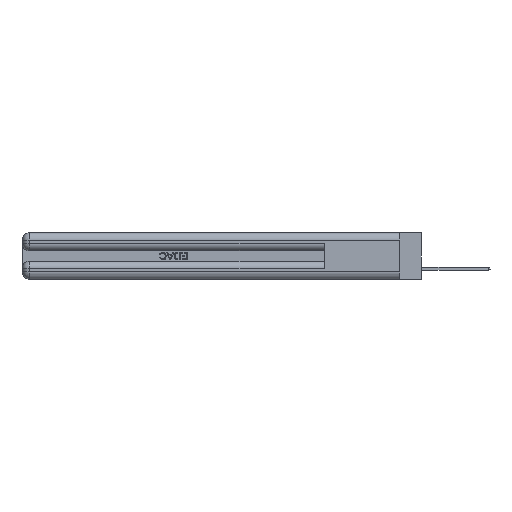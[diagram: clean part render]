
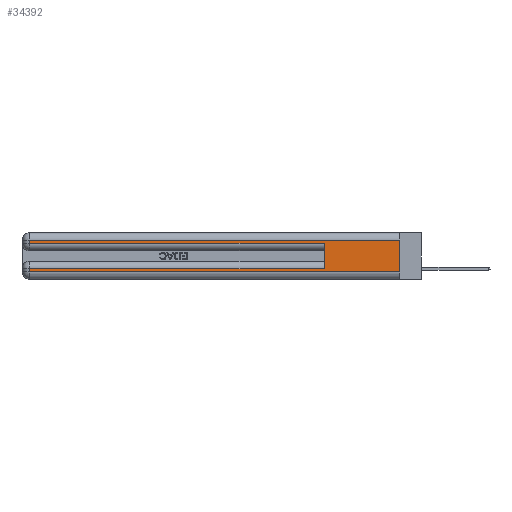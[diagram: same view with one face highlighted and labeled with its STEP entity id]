
A CAD part, left-side view. The second image highlights one B-rep face of the part: STEP entity #34392.
In plain terms, the highlighted planar face has unit normal (-1, 0, 0).
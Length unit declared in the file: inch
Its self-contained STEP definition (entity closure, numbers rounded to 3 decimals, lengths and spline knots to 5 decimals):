
#2489 = LINE ( 'NONE', #6364, #8938 ) ;
#2717 = VERTEX_POINT ( 'NONE', #44504 ) ;
#3348 = CARTESIAN_POINT ( 'NONE',  ( 0., 0.6, 0.085 ) ) ;
#4973 = CARTESIAN_POINT ( 'NONE',  ( 0., 2.94, 0.31 ) ) ;
#5919 = VECTOR ( 'NONE', #8321, 39.37008 ) ;
#6348 = ORIENTED_EDGE ( 'NONE', *, *, #17489, .T. ) ;
#6364 = CARTESIAN_POINT ( 'NONE',  ( 0., 0., 0.285 ) ) ;
#8077 = LINE ( 'NONE', #38608, #26345 ) ;
#8116 = CARTESIAN_POINT ( 'NONE',  ( 0., 0., 0.31 ) ) ;
#8321 = DIRECTION ( 'NONE',  ( 0., 0., 1. ) ) ;
#8938 = VECTOR ( 'NONE', #42705, 39.37008 ) ;
#9776 = LINE ( 'NONE', #14755, #48023 ) ;
#10958 = CARTESIAN_POINT ( 'NONE',  ( 0., 2.94, 0.085 ) ) ;
#11423 = LINE ( 'NONE', #25829, #29112 ) ;
#11937 = CARTESIAN_POINT ( 'NONE',  ( 0., 0.6, 0.145 ) ) ;
#12087 = PLANE ( 'NONE',  #47939 ) ;
#12150 = VERTEX_POINT ( 'NONE', #16853 ) ;
#12920 = DIRECTION ( 'NONE',  ( 0., 0., -1. ) ) ;
#13185 = EDGE_CURVE ( 'NONE', #21291, #37837, #46464, .T. ) ;
#13463 = CARTESIAN_POINT ( 'NONE',  ( 0., 0., 0.06 ) ) ;
#14755 = CARTESIAN_POINT ( 'NONE',  ( 0., 0., 0.37 ) ) ;
#15212 = CARTESIAN_POINT ( 'NONE',  ( 0., 0., 0.06 ) ) ;
#15460 = LINE ( 'NONE', #15524, #24281 ) ;
#15524 = CARTESIAN_POINT ( 'NONE',  ( 0., 0., 0.085 ) ) ;
#15884 = ORIENTED_EDGE ( 'NONE', *, *, #40547, .F. ) ;
#16217 = EDGE_CURVE ( 'NONE', #18066, #12150, #38505, .T. ) ;
#16572 = ORIENTED_EDGE ( 'NONE', *, *, #46242, .T. ) ;
#16853 = CARTESIAN_POINT ( 'NONE',  ( 0., 2.94, 0.06 ) ) ;
#17173 = ORIENTED_EDGE ( 'NONE', *, *, #16217, .T. ) ;
#17489 = EDGE_CURVE ( 'NONE', #2717, #37837, #2489, .T. ) ;
#18066 = VERTEX_POINT ( 'NONE', #10958 ) ;
#18533 = VECTOR ( 'NONE', #43790, 39.37008 ) ;
#21291 = VERTEX_POINT ( 'NONE', #3348 ) ;
#24074 = DIRECTION ( 'NONE',  ( 1., 0., 0. ) ) ;
#24281 = VECTOR ( 'NONE', #45780, 39.37008 ) ;
#24666 = ORIENTED_EDGE ( 'NONE', *, *, #13185, .F. ) ;
#25829 = CARTESIAN_POINT ( 'NONE',  ( 0., 2.94, 0.37 ) ) ;
#25979 = ORIENTED_EDGE ( 'NONE', *, *, #42214, .T. ) ;
#26345 = VECTOR ( 'NONE', #46168, 39.37008 ) ;
#27332 = CARTESIAN_POINT ( 'NONE',  ( 0., 0.6, 0.285 ) ) ;
#29112 = VECTOR ( 'NONE', #40987, 39.37008 ) ;
#31323 = CARTESIAN_POINT ( 'NONE',  ( 0., 0., 0.37 ) ) ;
#31707 = VECTOR ( 'NONE', #40107, 39.37008 ) ;
#32823 = FACE_OUTER_BOUND ( 'NONE', #36065, .T. ) ;
#34392 = ADVANCED_FACE ( 'NONE', ( #32823 ), #12087, .F. ) ;
#36065 = EDGE_LOOP ( 'NONE', ( #15884, #16572, #25979, #6348, #24666, #39979, #17173, #42682 ) ) ;
#37837 = VERTEX_POINT ( 'NONE', #27332 ) ;
#38505 = LINE ( 'NONE', #40325, #18533 ) ;
#38608 = CARTESIAN_POINT ( 'NONE',  ( 0., 0., 0.31 ) ) ;
#38876 = EDGE_CURVE ( 'NONE', #12150, #40754, #44711, .T. ) ;
#39979 = ORIENTED_EDGE ( 'NONE', *, *, #43553, .T. ) ;
#40107 = DIRECTION ( 'NONE',  ( 0., -1., 0. ) ) ;
#40325 = CARTESIAN_POINT ( 'NONE',  ( 0., 2.94, 0.37 ) ) ;
#40547 = EDGE_CURVE ( 'NONE', #44883, #40754, #9776, .T. ) ;
#40754 = VERTEX_POINT ( 'NONE', #15212 ) ;
#40987 = DIRECTION ( 'NONE',  ( 0., 0., -1. ) ) ;
#41912 = VERTEX_POINT ( 'NONE', #4973 ) ;
#42214 = EDGE_CURVE ( 'NONE', #41912, #2717, #11423, .T. ) ;
#42682 = ORIENTED_EDGE ( 'NONE', *, *, #38876, .T. ) ;
#42705 = DIRECTION ( 'NONE',  ( 0., -1., 0. ) ) ;
#43553 = EDGE_CURVE ( 'NONE', #21291, #18066, #15460, .T. ) ;
#43790 = DIRECTION ( 'NONE',  ( 0., 0., -1. ) ) ;
#44504 = CARTESIAN_POINT ( 'NONE',  ( 0., 2.94, 0.285 ) ) ;
#44693 = DIRECTION ( 'NONE',  ( 0., 0., -1. ) ) ;
#44711 = LINE ( 'NONE', #13463, #31707 ) ;
#44883 = VERTEX_POINT ( 'NONE', #8116 ) ;
#45780 = DIRECTION ( 'NONE',  ( 0., 1., 0. ) ) ;
#46168 = DIRECTION ( 'NONE',  ( 0., 1., 0. ) ) ;
#46242 = EDGE_CURVE ( 'NONE', #44883, #41912, #8077, .T. ) ;
#46464 = LINE ( 'NONE', #11937, #5919 ) ;
#47939 = AXIS2_PLACEMENT_3D ( 'NONE', #31323, #24074, #12920 ) ;
#48023 = VECTOR ( 'NONE', #44693, 39.37008 ) ;
